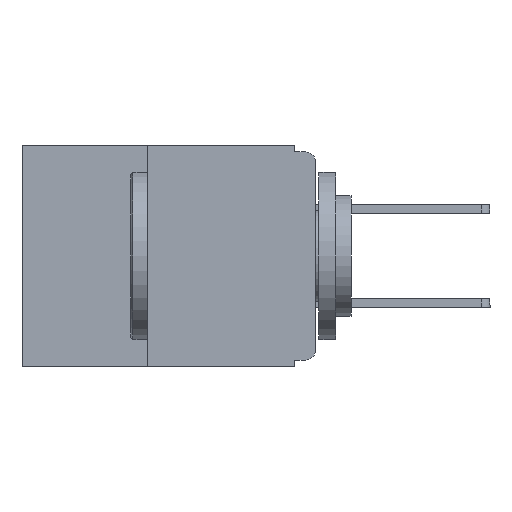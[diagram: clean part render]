
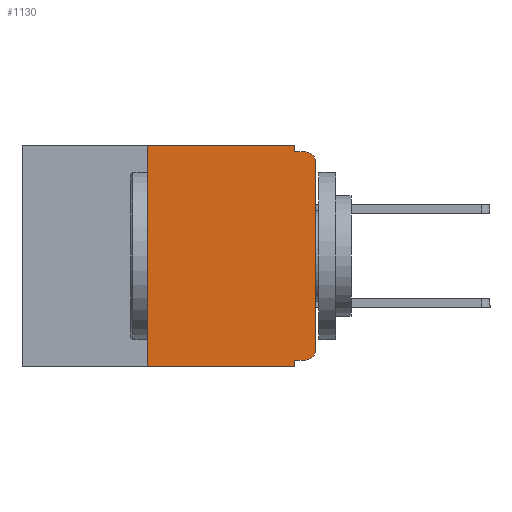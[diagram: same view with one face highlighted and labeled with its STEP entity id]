
A CAD part, left-side view. The second image highlights one B-rep face of the part: STEP entity #1130.
In plain terms, the highlighted planar face has unit normal (-1, 0, 0).
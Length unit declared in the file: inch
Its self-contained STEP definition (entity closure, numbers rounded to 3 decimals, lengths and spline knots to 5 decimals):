
#702 = VECTOR ( 'NONE', #17763, 39.37008 ) ;
#958 = CARTESIAN_POINT ( 'NONE',  ( 0., 0.031, -0.33 ) ) ;
#1130 = ADVANCED_FACE ( 'NONE', ( #19802 ), #24690, .F. ) ;
#1189 = ORIENTED_EDGE ( 'NONE', *, *, #8545, .T. ) ;
#1909 = DIRECTION ( 'NONE',  ( 0., -1., 0. ) ) ;
#2127 = VERTEX_POINT ( 'NONE', #34763 ) ;
#2407 = ORIENTED_EDGE ( 'NONE', *, *, #33348, .F. ) ;
#3143 = CARTESIAN_POINT ( 'NONE',  ( 0., 0.25, 0. ) ) ;
#4107 = CARTESIAN_POINT ( 'NONE',  ( 0., 0.031, -0.32 ) ) ;
#4244 = ORIENTED_EDGE ( 'NONE', *, *, #32124, .T. ) ;
#4587 = EDGE_LOOP ( 'NONE', ( #1189, #4244, #25707, #14916, #13325, #2407, #25126, #17019, #25480, #13287 ) ) ;
#4711 = CARTESIAN_POINT ( 'NONE',  ( 0., 0.015, -0.305 ) ) ;
#4724 = VERTEX_POINT ( 'NONE', #30430 ) ;
#4998 = CARTESIAN_POINT ( 'NONE',  ( 0., 0.031, -0.01 ) ) ;
#5150 = CARTESIAN_POINT ( 'NONE',  ( 0., 0.25, -0.33 ) ) ;
#5328 = LINE ( 'NONE', #26203, #28204 ) ;
#5476 = LINE ( 'NONE', #7486, #33795 ) ;
#6086 = VECTOR ( 'NONE', #34274, 39.37008 ) ;
#6762 = EDGE_CURVE ( 'NONE', #31149, #29817, #5328, .T. ) ;
#7486 = CARTESIAN_POINT ( 'NONE',  ( 0., 0.437, -0.33 ) ) ;
#7559 = DIRECTION ( 'NONE',  ( 0., 0., -1. ) ) ;
#7846 = CARTESIAN_POINT ( 'NONE',  ( 0., 0.25, -0.33 ) ) ;
#7953 = AXIS2_PLACEMENT_3D ( 'NONE', #4711, #24102, #7559 ) ;
#8545 = EDGE_CURVE ( 'NONE', #25577, #4724, #13510, .T. ) ;
#9744 = EDGE_CURVE ( 'NONE', #32953, #10733, #12623, .T. ) ;
#10733 = VERTEX_POINT ( 'NONE', #14672 ) ;
#11938 = DIRECTION ( 'NONE',  ( -1., 0., 0. ) ) ;
#12151 = CARTESIAN_POINT ( 'NONE',  ( 0., 0., -0.01 ) ) ;
#12623 = LINE ( 'NONE', #12151, #19950 ) ;
#12669 = LINE ( 'NONE', #30220, #25568 ) ;
#13287 = ORIENTED_EDGE ( 'NONE', *, *, #29283, .T. ) ;
#13325 = ORIENTED_EDGE ( 'NONE', *, *, #30648, .F. ) ;
#13510 = LINE ( 'NONE', #15325, #6086 ) ;
#14365 = AXIS2_PLACEMENT_3D ( 'NONE', #28364, #11938, #31098 ) ;
#14672 = CARTESIAN_POINT ( 'NONE',  ( 0., 0.015, -0.01 ) ) ;
#14901 = LINE ( 'NONE', #19109, #28556 ) ;
#14916 = ORIENTED_EDGE ( 'NONE', *, *, #26097, .F. ) ;
#15084 = CIRCLE ( 'NONE', #7953, 0.015 ) ;
#15325 = CARTESIAN_POINT ( 'NONE',  ( 0., 0., 0. ) ) ;
#17019 = ORIENTED_EDGE ( 'NONE', *, *, #26911, .F. ) ;
#17176 = VERTEX_POINT ( 'NONE', #3143 ) ;
#17763 = DIRECTION ( 'NONE',  ( 0., 0., -1. ) ) ;
#18141 = VERTEX_POINT ( 'NONE', #5150 ) ;
#19109 = CARTESIAN_POINT ( 'NONE',  ( 0., 0.031, 0. ) ) ;
#19158 = CARTESIAN_POINT ( 'NONE',  ( 0., 0.031, -0.33 ) ) ;
#19163 = VERTEX_POINT ( 'NONE', #19158 ) ;
#19802 = FACE_OUTER_BOUND ( 'NONE', #4587, .T. ) ;
#19950 = VECTOR ( 'NONE', #31191, 39.37008 ) ;
#21842 = DIRECTION ( 'NONE',  ( 0., 0., -1. ) ) ;
#22022 = DIRECTION ( 'NONE',  ( 0., -1., 0. ) ) ;
#24102 = DIRECTION ( 'NONE',  ( -1., 0., 0. ) ) ;
#24690 = PLANE ( 'NONE',  #25575 ) ;
#24903 = DIRECTION ( 'NONE',  ( 0., 1., 0. ) ) ;
#25126 = ORIENTED_EDGE ( 'NONE', *, *, #28708, .T. ) ;
#25480 = ORIENTED_EDGE ( 'NONE', *, *, #6762, .F. ) ;
#25568 = VECTOR ( 'NONE', #22022, 39.37008 ) ;
#25575 = AXIS2_PLACEMENT_3D ( 'NONE', #28956, #28913, #29778 ) ;
#25577 = VERTEX_POINT ( 'NONE', #27715 ) ;
#25707 = ORIENTED_EDGE ( 'NONE', *, *, #9744, .F. ) ;
#26097 = EDGE_CURVE ( 'NONE', #2127, #32953, #14901, .T. ) ;
#26203 = CARTESIAN_POINT ( 'NONE',  ( 0., 0., -0.32 ) ) ;
#26911 = EDGE_CURVE ( 'NONE', #29817, #19163, #31040, .T. ) ;
#27715 = CARTESIAN_POINT ( 'NONE',  ( 0., 0., -0.305 ) ) ;
#28204 = VECTOR ( 'NONE', #24903, 39.37008 ) ;
#28364 = CARTESIAN_POINT ( 'NONE',  ( 0., 0.015, -0.025 ) ) ;
#28556 = VECTOR ( 'NONE', #21842, 39.37008 ) ;
#28708 = EDGE_CURVE ( 'NONE', #18141, #19163, #5476, .T. ) ;
#28913 = DIRECTION ( 'NONE',  ( 1., 0., 0. ) ) ;
#28956 = CARTESIAN_POINT ( 'NONE',  ( 0., 0.437, 0. ) ) ;
#29144 = VECTOR ( 'NONE', #32537, 39.37008 ) ;
#29283 = EDGE_CURVE ( 'NONE', #31149, #25577, #15084, .T. ) ;
#29778 = DIRECTION ( 'NONE',  ( 0., 0., -1. ) ) ;
#29817 = VERTEX_POINT ( 'NONE', #4107 ) ;
#29976 = LINE ( 'NONE', #7846, #29144 ) ;
#30220 = CARTESIAN_POINT ( 'NONE',  ( 0., 0.437, 0. ) ) ;
#30430 = CARTESIAN_POINT ( 'NONE',  ( 0., 0., -0.025 ) ) ;
#30648 = EDGE_CURVE ( 'NONE', #17176, #2127, #12669, .T. ) ;
#31040 = LINE ( 'NONE', #958, #702 ) ;
#31098 = DIRECTION ( 'NONE',  ( 0., 0., -1. ) ) ;
#31149 = VERTEX_POINT ( 'NONE', #32298 ) ;
#31191 = DIRECTION ( 'NONE',  ( 0., -1., 0. ) ) ;
#32124 = EDGE_CURVE ( 'NONE', #4724, #10733, #33853, .T. ) ;
#32298 = CARTESIAN_POINT ( 'NONE',  ( 0., 0.015, -0.32 ) ) ;
#32537 = DIRECTION ( 'NONE',  ( 0., 0., 1. ) ) ;
#32953 = VERTEX_POINT ( 'NONE', #4998 ) ;
#33348 = EDGE_CURVE ( 'NONE', #18141, #17176, #29976, .T. ) ;
#33795 = VECTOR ( 'NONE', #1909, 39.37008 ) ;
#33853 = CIRCLE ( 'NONE', #14365, 0.015 ) ;
#34274 = DIRECTION ( 'NONE',  ( 0., 0., 1. ) ) ;
#34763 = CARTESIAN_POINT ( 'NONE',  ( 0., 0.031, 0. ) ) ;
